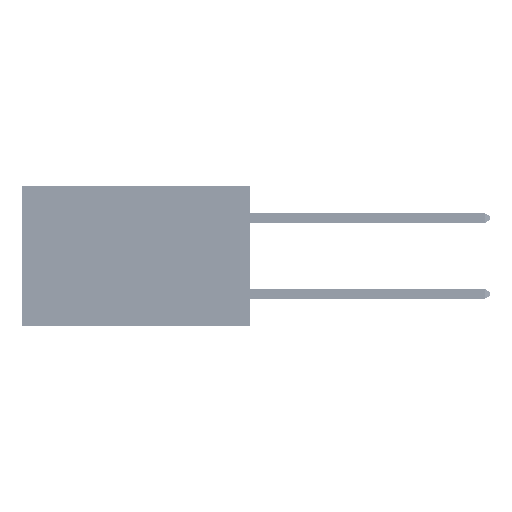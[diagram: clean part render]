
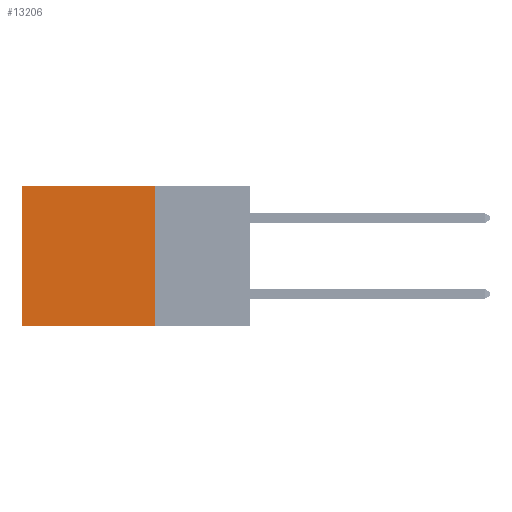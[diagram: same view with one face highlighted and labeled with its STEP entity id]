
A CAD part, left-side view. The second image highlights one B-rep face of the part: STEP entity #13206.
In plain terms, the highlighted planar face has unit normal (-1, 0, 0).
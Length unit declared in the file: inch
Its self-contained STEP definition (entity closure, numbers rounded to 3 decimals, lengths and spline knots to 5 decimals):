
#1930 = EDGE_CURVE ( 'NONE', #3864, #42571, #22932, .T. ) ;
#2191 = EDGE_CURVE ( 'NONE', #3864, #25479, #25804, .T. ) ;
#2333 = CARTESIAN_POINT ( 'NONE',  ( 0.2875, 0.25, 0. ) ) ;
#3864 = VERTEX_POINT ( 'NONE', #16265 ) ;
#4771 = CARTESIAN_POINT ( 'NONE',  ( 0.2875, 0.25, -0.37 ) ) ;
#5847 = VERTEX_POINT ( 'NONE', #33208 ) ;
#7823 = ORIENTED_EDGE ( 'NONE', *, *, #18080, .F. ) ;
#10145 = PLANE ( 'NONE',  #40921 ) ;
#10470 = CARTESIAN_POINT ( 'NONE',  ( 0.2875, 0.25, 0. ) ) ;
#10710 = CARTESIAN_POINT ( 'NONE',  ( 0.2875, 0.6, 0. ) ) ;
#11331 = VECTOR ( 'NONE', #38972, 39.37008 ) ;
#13206 = ADVANCED_FACE ( 'NONE', ( #21932 ), #10145, .F. ) ;
#14521 = EDGE_CURVE ( 'NONE', #42571, #5847, #19171, .T. ) ;
#16265 = CARTESIAN_POINT ( 'NONE',  ( 0.2875, 0.25, 0. ) ) ;
#17124 = VECTOR ( 'NONE', #51980, 39.37008 ) ;
#18080 = EDGE_CURVE ( 'NONE', #25479, #5847, #49620, .T. ) ;
#19171 = LINE ( 'NONE', #51481, #47075 ) ;
#19364 = DIRECTION ( 'NONE',  ( 0., 0., -1. ) ) ;
#20635 = VECTOR ( 'NONE', #21642, 39.37008 ) ;
#21352 = EDGE_LOOP ( 'NONE', ( #28154, #7823, #48549, #31356 ) ) ;
#21642 = DIRECTION ( 'NONE',  ( 0., 0., -1. ) ) ;
#21932 = FACE_OUTER_BOUND ( 'NONE', #21352, .T. ) ;
#22631 = DIRECTION ( 'NONE',  ( 1., 0., 0. ) ) ;
#22641 = DIRECTION ( 'NONE',  ( 0., 0., -1. ) ) ;
#22932 = LINE ( 'NONE', #10470, #17124 ) ;
#25479 = VERTEX_POINT ( 'NONE', #4771 ) ;
#25804 = LINE ( 'NONE', #41422, #20635 ) ;
#28154 = ORIENTED_EDGE ( 'NONE', *, *, #14521, .T. ) ;
#30232 = CARTESIAN_POINT ( 'NONE',  ( 0.2875, 0.25, -0.37 ) ) ;
#31356 = ORIENTED_EDGE ( 'NONE', *, *, #1930, .T. ) ;
#33208 = CARTESIAN_POINT ( 'NONE',  ( 0.2875, 0.6, -0.37 ) ) ;
#38972 = DIRECTION ( 'NONE',  ( 0., 1., 0. ) ) ;
#40921 = AXIS2_PLACEMENT_3D ( 'NONE', #2333, #22631, #19364 ) ;
#41422 = CARTESIAN_POINT ( 'NONE',  ( 0.2875, 0.25, 0. ) ) ;
#42571 = VERTEX_POINT ( 'NONE', #10710 ) ;
#47075 = VECTOR ( 'NONE', #22641, 39.37008 ) ;
#48549 = ORIENTED_EDGE ( 'NONE', *, *, #2191, .F. ) ;
#49620 = LINE ( 'NONE', #30232, #11331 ) ;
#51481 = CARTESIAN_POINT ( 'NONE',  ( 0.2875, 0.6, 0. ) ) ;
#51980 = DIRECTION ( 'NONE',  ( 0., 1., 0. ) ) ;
